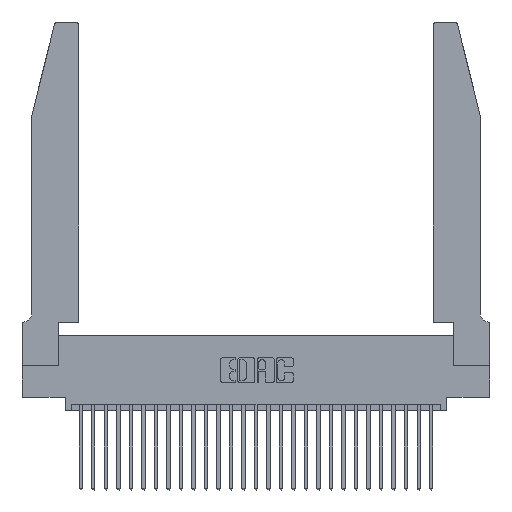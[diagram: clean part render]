
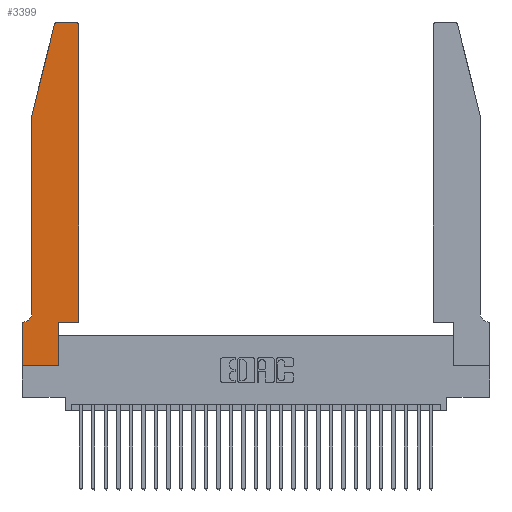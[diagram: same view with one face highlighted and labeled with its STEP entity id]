
A CAD part, top view. The second image highlights one B-rep face of the part: STEP entity #3399.
In plain terms, the highlighted planar face has unit normal (0, 0, 1).
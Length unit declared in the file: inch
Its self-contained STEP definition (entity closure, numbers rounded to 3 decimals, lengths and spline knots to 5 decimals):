
#120 = CARTESIAN_POINT ( 'NONE',  ( 0.2865, 0., 0.37 ) ) ;
#500 = ORIENTED_EDGE ( 'NONE', *, *, #3964, .T. ) ;
#1182 = VECTOR ( 'NONE', #16583, 39.37008 ) ;
#1402 = VECTOR ( 'NONE', #27520, 39.37008 ) ;
#1973 = DIRECTION ( 'NONE',  ( 0., -1., 0. ) ) ;
#2201 = CIRCLE ( 'NONE', #17170, 0.03 ) ;
#2343 = DIRECTION ( 'NONE',  ( 0., 1., 0. ) ) ;
#2892 = VECTOR ( 'NONE', #1973, 39.37008 ) ;
#2962 = DIRECTION ( 'NONE',  ( -1., 0., 0. ) ) ;
#3399 = ADVANCED_FACE ( 'NONE', ( #4355 ), #4834, .T. ) ;
#3831 = LINE ( 'NONE', #17868, #15988 ) ;
#3964 = EDGE_CURVE ( 'NONE', #24751, #16468, #27088, .T. ) ;
#4067 = VERTEX_POINT ( 'NONE', #5225 ) ;
#4155 = DIRECTION ( 'NONE',  ( 0., 1., 0. ) ) ;
#4208 = DIRECTION ( 'NONE',  ( 0., -1., 0. ) ) ;
#4355 = FACE_OUTER_BOUND ( 'NONE', #4980, .T. ) ;
#4385 = EDGE_CURVE ( 'NONE', #18430, #8930, #27058, .T. ) ;
#4809 = CARTESIAN_POINT ( 'NONE',  ( 0.0755, 2., 0.37 ) ) ;
#4834 = PLANE ( 'NONE',  #4928 ) ;
#4928 = AXIS2_PLACEMENT_3D ( 'NONE', #9458, #25301, #11752 ) ;
#4980 = EDGE_LOOP ( 'NONE', ( #25091, #8739, #500, #7310, #7404, #6492, #15275, #23527, #5981, #11402, #27404, #21754 ) ) ;
#5201 = VERTEX_POINT ( 'NONE', #7084 ) ;
#5225 = CARTESIAN_POINT ( 'NONE',  ( 0.0055, 0.35, 0.37 ) ) ;
#5533 = VERTEX_POINT ( 'NONE', #19443 ) ;
#5971 = DIRECTION ( 'NONE',  ( 0., 0., 1. ) ) ;
#5981 = ORIENTED_EDGE ( 'NONE', *, *, #8255, .T. ) ;
#6121 = CARTESIAN_POINT ( 'NONE',  ( 0.4205, 2.72, 0.37 ) ) ;
#6278 = CARTESIAN_POINT ( 'NONE',  ( 0.4205, 2.75, 0.37 ) ) ;
#6492 = ORIENTED_EDGE ( 'NONE', *, *, #15068, .T. ) ;
#6920 = LINE ( 'NONE', #15691, #2892 ) ;
#7084 = CARTESIAN_POINT ( 'NONE',  ( 0., 0.35, 0.37 ) ) ;
#7140 = VERTEX_POINT ( 'NONE', #21214 ) ;
#7310 = ORIENTED_EDGE ( 'NONE', *, *, #16692, .T. ) ;
#7358 = CARTESIAN_POINT ( 'NONE',  ( 0.4505, 0.35, 0.37 ) ) ;
#7404 = ORIENTED_EDGE ( 'NONE', *, *, #13077, .T. ) ;
#7667 = LINE ( 'NONE', #8820, #13702 ) ;
#8255 = EDGE_CURVE ( 'NONE', #8930, #7140, #10536, .T. ) ;
#8441 = DIRECTION ( 'NONE',  ( 1., 0., 0. ) ) ;
#8739 = ORIENTED_EDGE ( 'NONE', *, *, #25733, .T. ) ;
#8815 = DIRECTION ( 'NONE',  ( 1., 0., 0. ) ) ;
#8820 = CARTESIAN_POINT ( 'NONE',  ( 0.4505, 0.35, 0.37 ) ) ;
#8886 = VECTOR ( 'NONE', #2962, 39.37008 ) ;
#8930 = VERTEX_POINT ( 'NONE', #120 ) ;
#9458 = CARTESIAN_POINT ( 'NONE',  ( 0., 0.35, 0.37 ) ) ;
#9491 = EDGE_CURVE ( 'NONE', #27479, #5533, #7667, .T. ) ;
#9644 = DIRECTION ( 'NONE',  ( 1., 0., 0. ) ) ;
#9797 = CARTESIAN_POINT ( 'NONE',  ( 0.284, 2.75, 0.37 ) ) ;
#9818 = VECTOR ( 'NONE', #2343, 39.37008 ) ;
#9910 = AXIS2_PLACEMENT_3D ( 'NONE', #13395, #29109, #15630 ) ;
#10536 = LINE ( 'NONE', #13809, #9818 ) ;
#10917 = EDGE_CURVE ( 'NONE', #7140, #27479, #24252, .T. ) ;
#11204 = EDGE_CURVE ( 'NONE', #5533, #22486, #18528, .T. ) ;
#11402 = ORIENTED_EDGE ( 'NONE', *, *, #10917, .T. ) ;
#11752 = DIRECTION ( 'NONE',  ( 1., 0., 0. ) ) ;
#12137 = CARTESIAN_POINT ( 'NONE',  ( 0.2605, 2.75, 0.37 ) ) ;
#12671 = CARTESIAN_POINT ( 'NONE',  ( 0.0755, 2., 0.37 ) ) ;
#13077 = EDGE_CURVE ( 'NONE', #27565, #4067, #22714, .T. ) ;
#13297 = CARTESIAN_POINT ( 'NONE',  ( 0.4505, 0.35, 0.37 ) ) ;
#13395 = CARTESIAN_POINT ( 'NONE',  ( 0.0055, 0.42, 0.37 ) ) ;
#13490 = CARTESIAN_POINT ( 'NONE',  ( 0.0755, 0.42, 0.37 ) ) ;
#13702 = VECTOR ( 'NONE', #4155, 39.37008 ) ;
#13809 = CARTESIAN_POINT ( 'NONE',  ( 0.2865, 0.35, 0.37 ) ) ;
#14229 = LINE ( 'NONE', #12137, #8886 ) ;
#15068 = EDGE_CURVE ( 'NONE', #4067, #5201, #19427, .T. ) ;
#15150 = CARTESIAN_POINT ( 'NONE',  ( 0., 0., 0.37 ) ) ;
#15275 = ORIENTED_EDGE ( 'NONE', *, *, #28591, .T. ) ;
#15358 = CARTESIAN_POINT ( 'NONE',  ( 0.25487, 2.72718, 0.37 ) ) ;
#15630 = DIRECTION ( 'NONE',  ( -1., 0., 0. ) ) ;
#15691 = CARTESIAN_POINT ( 'NONE',  ( 0.0755, 2., 0.37 ) ) ;
#15988 = VECTOR ( 'NONE', #4208, 39.37008 ) ;
#16290 = VERTEX_POINT ( 'NONE', #9797 ) ;
#16468 = VERTEX_POINT ( 'NONE', #12671 ) ;
#16583 = DIRECTION ( 'NONE',  ( -1., 0., 0. ) ) ;
#16692 = EDGE_CURVE ( 'NONE', #16468, #27565, #6920, .T. ) ;
#17170 = AXIS2_PLACEMENT_3D ( 'NONE', #19586, #5971, #21883 ) ;
#17868 = CARTESIAN_POINT ( 'NONE',  ( 0., 0., 0.37 ) ) ;
#18194 = VECTOR ( 'NONE', #9644, 39.37008 ) ;
#18430 = VERTEX_POINT ( 'NONE', #18522 ) ;
#18522 = CARTESIAN_POINT ( 'NONE',  ( 0., 0., 0.37 ) ) ;
#18528 = CIRCLE ( 'NONE', #19355, 0.03 ) ;
#19355 = AXIS2_PLACEMENT_3D ( 'NONE', #6121, #22034, #8441 ) ;
#19427 = LINE ( 'NONE', #27830, #1182 ) ;
#19443 = CARTESIAN_POINT ( 'NONE',  ( 0.4505, 2.72, 0.37 ) ) ;
#19586 = CARTESIAN_POINT ( 'NONE',  ( 0.284, 2.72, 0.37 ) ) ;
#21072 = VECTOR ( 'NONE', #8815, 39.37008 ) ;
#21214 = CARTESIAN_POINT ( 'NONE',  ( 0.2865, 0.35, 0.37 ) ) ;
#21754 = ORIENTED_EDGE ( 'NONE', *, *, #11204, .T. ) ;
#21883 = DIRECTION ( 'NONE',  ( 1., 0., 0. ) ) ;
#22034 = DIRECTION ( 'NONE',  ( 0., 0., 1. ) ) ;
#22486 = VERTEX_POINT ( 'NONE', #6278 ) ;
#22714 = CIRCLE ( 'NONE', #9910, 0.07 ) ;
#23378 = EDGE_CURVE ( 'NONE', #22486, #16290, #14229, .T. ) ;
#23527 = ORIENTED_EDGE ( 'NONE', *, *, #4385, .T. ) ;
#24252 = LINE ( 'NONE', #7358, #18194 ) ;
#24751 = VERTEX_POINT ( 'NONE', #15358 ) ;
#25091 = ORIENTED_EDGE ( 'NONE', *, *, #23378, .T. ) ;
#25301 = DIRECTION ( 'NONE',  ( 0., 0., 1. ) ) ;
#25733 = EDGE_CURVE ( 'NONE', #16290, #24751, #2201, .T. ) ;
#27058 = LINE ( 'NONE', #15150, #21072 ) ;
#27088 = LINE ( 'NONE', #4809, #1402 ) ;
#27404 = ORIENTED_EDGE ( 'NONE', *, *, #9491, .T. ) ;
#27479 = VERTEX_POINT ( 'NONE', #13297 ) ;
#27520 = DIRECTION ( 'NONE',  ( -0.239, -0.971, 0. ) ) ;
#27565 = VERTEX_POINT ( 'NONE', #13490 ) ;
#27830 = CARTESIAN_POINT ( 'NONE',  ( 0.0755, 0.35, 0.37 ) ) ;
#28591 = EDGE_CURVE ( 'NONE', #5201, #18430, #3831, .T. ) ;
#29109 = DIRECTION ( 'NONE',  ( 0., 0., -1. ) ) ;
